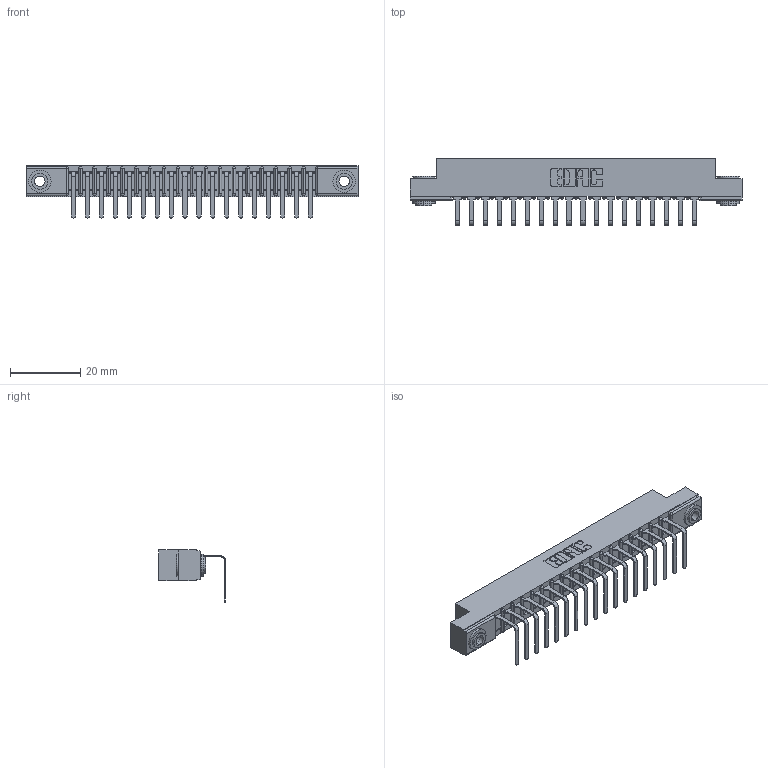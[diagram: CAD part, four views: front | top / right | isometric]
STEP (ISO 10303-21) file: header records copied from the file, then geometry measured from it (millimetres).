
FILE_DESCRIPTION (( 'STEP AP203' ), '1' );
FILE_NAME ('307-018-558-103.STEP', '2019-09-04T13:01:56', ( '' ), ( '' ), 'SwSTEP 2.0', 'SolidWorks 2016', '' );
FILE_SCHEMA (( 'CONFIG_CONTROL_DESIGN' ));
Length unit declared in the file: inch
Products named in the file (4): 307 Part_.156 Dia Mounting Holes; 345-250-002_345-250-002-102; 307-018-558-103; 307-290-001_558 - 2 (Single)
Assembly tree (21 placements, depth 2):
  307-018-558-103
    307 Part_.156 Dia Mounting Holes
    307-290-001_558 - 2 (Single)  x18
    345-250-002_345-250-002-102  x2
Bounding box: 94.34 x 18.96 x 14.81 mm (x, y, z)
Volume: 6048.9 mm3; surface area: 9974.3 mm2
Topology: 21 solids, 21 shells, 1269 faces, 3567 edges, 2298 vertices
Faces by surface type: plane 796, cylinder 427, sphere 38, cone 8
Entity records: 19559 total; most frequent: CARTESIAN_POINT 3265, ORIENTED_EDGE 3242, DIRECTION 3205, EDGE_CURVE 1621, LINE 1225, VECTOR 1225, VERTEX_POINT 1050, AXIS2_PLACEMENT_3D 990
